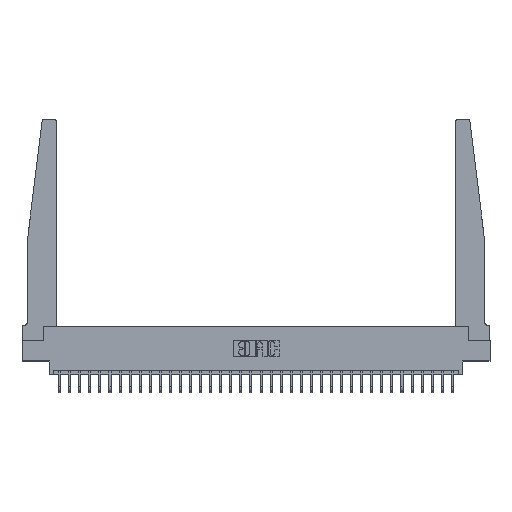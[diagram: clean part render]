
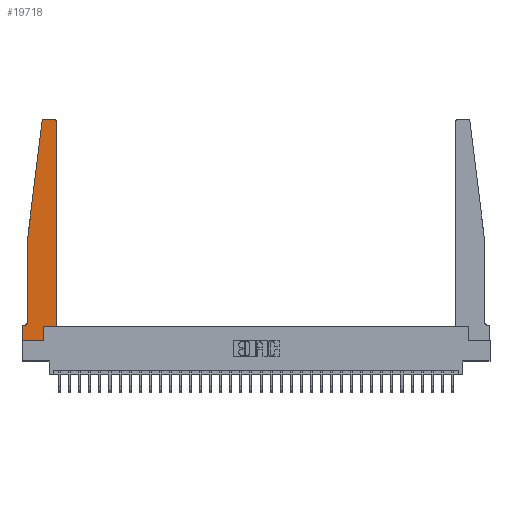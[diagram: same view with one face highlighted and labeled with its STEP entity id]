
A CAD part, top view. The second image highlights one B-rep face of the part: STEP entity #19718.
In plain terms, the highlighted planar face has unit normal (0, 0, 1).
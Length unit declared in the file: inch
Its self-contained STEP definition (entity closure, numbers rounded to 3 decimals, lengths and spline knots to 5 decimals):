
#453 = CARTESIAN_POINT ( 'NONE',  ( 0.425, 0.18, 0.37 ) ) ;
#668 = DIRECTION ( 'NONE',  ( 0., 1., 0. ) ) ;
#936 = DIRECTION ( 'NONE',  ( -0.122, -0.992, 0. ) ) ;
#1191 = CARTESIAN_POINT ( 'NONE',  ( 0.25, 2.75, 0.37 ) ) ;
#1932 = EDGE_LOOP ( 'NONE', ( #6153, #23204, #4098, #15865, #4693, #18251, #22978, #20798, #16744, #29697, #21899, #15327 ) ) ;
#2528 = VECTOR ( 'NONE', #12800, 39.37008 ) ;
#3176 = CARTESIAN_POINT ( 'NONE',  ( 0.2605, 0.18, 0.37 ) ) ;
#3936 = CARTESIAN_POINT ( 'NONE',  ( 0.395, 2.72, 0.37 ) ) ;
#4010 = VECTOR ( 'NONE', #28090, 39.37008 ) ;
#4069 = PLANE ( 'NONE',  #19751 ) ;
#4098 = ORIENTED_EDGE ( 'NONE', *, *, #29983, .T. ) ;
#4256 = VECTOR ( 'NONE', #8472, 39.37008 ) ;
#4693 = ORIENTED_EDGE ( 'NONE', *, *, #13471, .T. ) ;
#4774 = CARTESIAN_POINT ( 'NONE',  ( 0., 0.1875, 0.37 ) ) ;
#4787 = LINE ( 'NONE', #20003, #16401 ) ;
#4952 = CARTESIAN_POINT ( 'NONE',  ( 0.27653, 2.72, 0.37 ) ) ;
#5204 = LINE ( 'NONE', #15724, #31953 ) ;
#5392 = VERTEX_POINT ( 'NONE', #27273 ) ;
#5507 = LINE ( 'NONE', #3176, #9996 ) ;
#5530 = CARTESIAN_POINT ( 'NONE',  ( 0.425, 0.18, 0.37 ) ) ;
#6153 = ORIENTED_EDGE ( 'NONE', *, *, #11611, .T. ) ;
#6496 = CARTESIAN_POINT ( 'NONE',  ( 0.065, 1.25, 0.37 ) ) ;
#6740 = CARTESIAN_POINT ( 'NONE',  ( 0., 0.1875, 0.37 ) ) ;
#7090 = EDGE_CURVE ( 'NONE', #12523, #13585, #5204, .T. ) ;
#7120 = CARTESIAN_POINT ( 'NONE',  ( 0.24675, 2.72367, 0.37 ) ) ;
#7188 = EDGE_CURVE ( 'NONE', #19542, #27182, #4787, .T. ) ;
#7379 = LINE ( 'NONE', #22968, #2528 ) ;
#8114 = VERTEX_POINT ( 'NONE', #21948 ) ;
#8472 = DIRECTION ( 'NONE',  ( 1., 0., 0. ) ) ;
#9152 = DIRECTION ( 'NONE',  ( 1., 0., 0. ) ) ;
#9337 = EDGE_CURVE ( 'NONE', #20047, #19542, #15065, .T. ) ;
#9609 = DIRECTION ( 'NONE',  ( 0., 0., 1. ) ) ;
#9734 = CARTESIAN_POINT ( 'NONE',  ( 0.065, 0.2375, 0.37 ) ) ;
#9767 = CIRCLE ( 'NONE', #20475, 0.03 ) ;
#9996 = VECTOR ( 'NONE', #668, 39.37008 ) ;
#10004 = EDGE_CURVE ( 'NONE', #5392, #32487, #26632, .T. ) ;
#11184 = CARTESIAN_POINT ( 'NONE',  ( 0.065, 1.25, 0.37 ) ) ;
#11291 = EDGE_CURVE ( 'NONE', #28617, #20047, #26059, .T. ) ;
#11476 = VERTEX_POINT ( 'NONE', #24495 ) ;
#11611 = EDGE_CURVE ( 'NONE', #11476, #8114, #29571, .T. ) ;
#12523 = VERTEX_POINT ( 'NONE', #6496 ) ;
#12540 = DIRECTION ( 'NONE',  ( -1., 0., 0. ) ) ;
#12800 = DIRECTION ( 'NONE',  ( 0., 1., 0. ) ) ;
#13020 = LINE ( 'NONE', #11184, #28589 ) ;
#13471 = EDGE_CURVE ( 'NONE', #13585, #28617, #25899, .T. ) ;
#13585 = VERTEX_POINT ( 'NONE', #9734 ) ;
#14016 = VECTOR ( 'NONE', #31703, 39.37008 ) ;
#14360 = VERTEX_POINT ( 'NONE', #7120 ) ;
#15065 = LINE ( 'NONE', #27350, #33012 ) ;
#15263 = EDGE_CURVE ( 'NONE', #32487, #16553, #7379, .T. ) ;
#15327 = ORIENTED_EDGE ( 'NONE', *, *, #24932, .T. ) ;
#15587 = CARTESIAN_POINT ( 'NONE',  ( 0.2605, 0., 0.37 ) ) ;
#15724 = CARTESIAN_POINT ( 'NONE',  ( 0.065, 1.25, 0.37 ) ) ;
#15865 = ORIENTED_EDGE ( 'NONE', *, *, #7090, .T. ) ;
#16401 = VECTOR ( 'NONE', #27463, 39.37008 ) ;
#16553 = VERTEX_POINT ( 'NONE', #25265 ) ;
#16744 = ORIENTED_EDGE ( 'NONE', *, *, #23178, .T. ) ;
#17730 = DIRECTION ( 'NONE',  ( 1., 0., 0. ) ) ;
#18251 = ORIENTED_EDGE ( 'NONE', *, *, #11291, .T. ) ;
#19542 = VERTEX_POINT ( 'NONE', #30788 ) ;
#19718 = ADVANCED_FACE ( 'NONE', ( #22959 ), #4069, .T. ) ;
#19751 = AXIS2_PLACEMENT_3D ( 'NONE', #6740, #27247, #29768 ) ;
#19760 = DIRECTION ( 'NONE',  ( 0., -1., 0. ) ) ;
#20003 = CARTESIAN_POINT ( 'NONE',  ( 0., 0., 0.37 ) ) ;
#20047 = VERTEX_POINT ( 'NONE', #4774 ) ;
#20206 = EDGE_CURVE ( 'NONE', #8114, #14360, #9767, .T. ) ;
#20441 = DIRECTION ( 'NONE',  ( 0., 0., 1. ) ) ;
#20475 = AXIS2_PLACEMENT_3D ( 'NONE', #4952, #20441, #17730 ) ;
#20545 = CIRCLE ( 'NONE', #26522, 0.03 ) ;
#20798 = ORIENTED_EDGE ( 'NONE', *, *, #7188, .T. ) ;
#21899 = ORIENTED_EDGE ( 'NONE', *, *, #15263, .T. ) ;
#21948 = CARTESIAN_POINT ( 'NONE',  ( 0.27653, 2.75, 0.37 ) ) ;
#22959 = FACE_OUTER_BOUND ( 'NONE', #1932, .T. ) ;
#22968 = CARTESIAN_POINT ( 'NONE',  ( 0.425, 0.18, 0.37 ) ) ;
#22978 = ORIENTED_EDGE ( 'NONE', *, *, #9337, .T. ) ;
#23178 = EDGE_CURVE ( 'NONE', #27182, #5392, #5507, .T. ) ;
#23204 = ORIENTED_EDGE ( 'NONE', *, *, #20206, .T. ) ;
#24325 = AXIS2_PLACEMENT_3D ( 'NONE', #30053, #25289, #12540 ) ;
#24495 = CARTESIAN_POINT ( 'NONE',  ( 0.395, 2.75, 0.37 ) ) ;
#24932 = EDGE_CURVE ( 'NONE', #16553, #11476, #20545, .T. ) ;
#25265 = CARTESIAN_POINT ( 'NONE',  ( 0.425, 2.72, 0.37 ) ) ;
#25289 = DIRECTION ( 'NONE',  ( 0., 0., -1. ) ) ;
#25899 = CIRCLE ( 'NONE', #24325, 0.05 ) ;
#26059 = LINE ( 'NONE', #30438, #4010 ) ;
#26522 = AXIS2_PLACEMENT_3D ( 'NONE', #3936, #9609, #9152 ) ;
#26632 = LINE ( 'NONE', #453, #4256 ) ;
#27182 = VERTEX_POINT ( 'NONE', #15587 ) ;
#27247 = DIRECTION ( 'NONE',  ( 0., 0., 1. ) ) ;
#27273 = CARTESIAN_POINT ( 'NONE',  ( 0.2605, 0.18, 0.37 ) ) ;
#27350 = CARTESIAN_POINT ( 'NONE',  ( 0., 0., 0.37 ) ) ;
#27463 = DIRECTION ( 'NONE',  ( 1., 0., 0. ) ) ;
#28090 = DIRECTION ( 'NONE',  ( -1., 0., 0. ) ) ;
#28589 = VECTOR ( 'NONE', #936, 39.37008 ) ;
#28617 = VERTEX_POINT ( 'NONE', #31006 ) ;
#29571 = LINE ( 'NONE', #1191, #14016 ) ;
#29697 = ORIENTED_EDGE ( 'NONE', *, *, #10004, .T. ) ;
#29768 = DIRECTION ( 'NONE',  ( 1., 0., 0. ) ) ;
#29983 = EDGE_CURVE ( 'NONE', #14360, #12523, #13020, .T. ) ;
#30053 = CARTESIAN_POINT ( 'NONE',  ( 0.015, 0.2375, 0.37 ) ) ;
#30438 = CARTESIAN_POINT ( 'NONE',  ( 0.065, 0.1875, 0.37 ) ) ;
#30788 = CARTESIAN_POINT ( 'NONE',  ( 0., 0., 0.37 ) ) ;
#30889 = DIRECTION ( 'NONE',  ( 0., -1., 0. ) ) ;
#31006 = CARTESIAN_POINT ( 'NONE',  ( 0.015, 0.1875, 0.37 ) ) ;
#31703 = DIRECTION ( 'NONE',  ( -1., 0., 0. ) ) ;
#31953 = VECTOR ( 'NONE', #30889, 39.37008 ) ;
#32487 = VERTEX_POINT ( 'NONE', #5530 ) ;
#33012 = VECTOR ( 'NONE', #19760, 39.37008 ) ;
